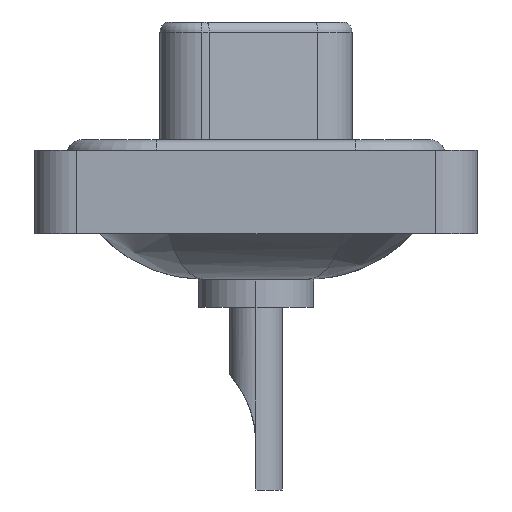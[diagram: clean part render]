
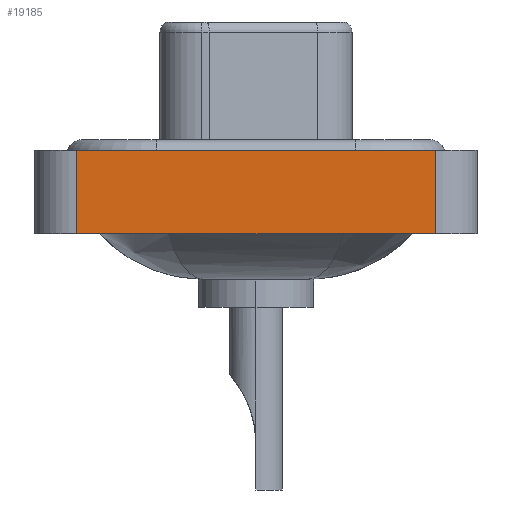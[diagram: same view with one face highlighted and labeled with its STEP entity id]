
A CAD part, left-side view. The second image highlights one B-rep face of the part: STEP entity #19185.
In plain terms, the highlighted planar face has unit normal (-1, 0, 0).
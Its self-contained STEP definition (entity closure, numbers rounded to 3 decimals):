
#943 = VERTEX_POINT ( 'NONE', #2029 ) ;
#2029 = CARTESIAN_POINT ( 'NONE',  ( -7.3, 8.55, 0.4 ) ) ;
#2896 = DIRECTION ( 'NONE',  ( 0., 0., 1. ) ) ;
#3051 = EDGE_CURVE ( 'NONE', #5391, #943, #11189, .T. ) ;
#3056 = VECTOR ( 'NONE', #10990, 1000. ) ;
#4159 = PLANE ( 'NONE',  #8047 ) ;
#4843 = EDGE_CURVE ( 'NONE', #943, #6541, #14187, .T. ) ;
#5205 = DIRECTION ( 'NONE',  ( 0., -1., 0. ) ) ;
#5391 = VERTEX_POINT ( 'NONE', #14157 ) ;
#5619 = ORIENTED_EDGE ( 'NONE', *, *, #11731, .T. ) ;
#6199 = CARTESIAN_POINT ( 'NONE',  ( -7.3, -8.55, -3.6 ) ) ;
#6541 = VERTEX_POINT ( 'NONE', #8512 ) ;
#6773 = DIRECTION ( 'NONE',  ( -1., 0., 0. ) ) ;
#6976 = CARTESIAN_POINT ( 'NONE',  ( -7.3, -8.55, -3.6 ) ) ;
#7324 = VECTOR ( 'NONE', #2896, 1000. ) ;
#8047 = AXIS2_PLACEMENT_3D ( 'NONE', #6976, #6773, #9870 ) ;
#8309 = VERTEX_POINT ( 'NONE', #19260 ) ;
#8508 = LINE ( 'NONE', #19039, #16151 ) ;
#8512 = CARTESIAN_POINT ( 'NONE',  ( -7.3, -8.55, 0.4 ) ) ;
#9870 = DIRECTION ( 'NONE',  ( 0., 0., 1. ) ) ;
#10595 = LINE ( 'NONE', #6199, #7324 ) ;
#10623 = ORIENTED_EDGE ( 'NONE', *, *, #3051, .F. ) ;
#10990 = DIRECTION ( 'NONE',  ( 0., 0., 1. ) ) ;
#11189 = LINE ( 'NONE', #18611, #3056 ) ;
#11731 = EDGE_CURVE ( 'NONE', #5391, #8309, #8508, .T. ) ;
#14157 = CARTESIAN_POINT ( 'NONE',  ( -7.3, 8.55, -3.6 ) ) ;
#14187 = LINE ( 'NONE', #17205, #15439 ) ;
#14516 = ORIENTED_EDGE ( 'NONE', *, *, #16906, .T. ) ;
#15439 = VECTOR ( 'NONE', #19744, 1000. ) ;
#16123 = ORIENTED_EDGE ( 'NONE', *, *, #4843, .F. ) ;
#16151 = VECTOR ( 'NONE', #5205, 1000. ) ;
#16906 = EDGE_CURVE ( 'NONE', #8309, #6541, #10595, .T. ) ;
#17205 = CARTESIAN_POINT ( 'NONE',  ( -7.3, -8.55, 0.4 ) ) ;
#17813 = EDGE_LOOP ( 'NONE', ( #14516, #16123, #10623, #5619 ) ) ;
#18611 = CARTESIAN_POINT ( 'NONE',  ( -7.3, 8.55, -3.6 ) ) ;
#19039 = CARTESIAN_POINT ( 'NONE',  ( -7.3, -8.55, -3.6 ) ) ;
#19096 = FACE_OUTER_BOUND ( 'NONE', #17813, .T. ) ;
#19185 = ADVANCED_FACE ( 'NONE', ( #19096 ), #4159, .T. ) ;
#19260 = CARTESIAN_POINT ( 'NONE',  ( -7.3, -8.55, -3.6 ) ) ;
#19744 = DIRECTION ( 'NONE',  ( 0., -1., 0. ) ) ;
